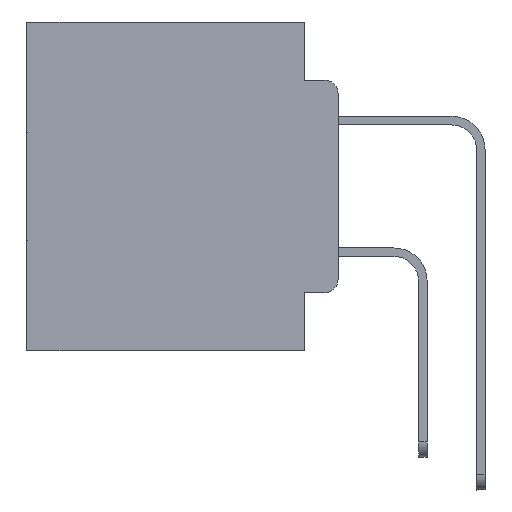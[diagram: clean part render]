
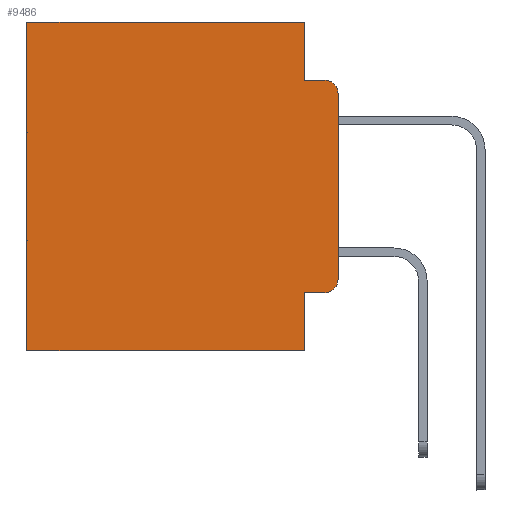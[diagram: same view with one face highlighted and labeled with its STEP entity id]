
A CAD part, left-side view. The second image highlights one B-rep face of the part: STEP entity #9486.
In plain terms, the highlighted planar face has unit normal (-1, 0, 0).
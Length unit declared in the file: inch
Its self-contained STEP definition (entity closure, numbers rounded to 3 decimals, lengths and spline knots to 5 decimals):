
#367 = VERTEX_POINT ( 'NONE', #19383 ) ;
#845 = EDGE_CURVE ( 'NONE', #2925, #9180, #17679, .T. ) ;
#854 = EDGE_CURVE ( 'NONE', #32254, #20370, #29934, .T. ) ;
#862 = LINE ( 'NONE', #9563, #12918 ) ;
#892 = VERTEX_POINT ( 'NONE', #26301 ) ;
#1207 = VECTOR ( 'NONE', #10588, 39.37008 ) ;
#1329 = ORIENTED_EDGE ( 'NONE', *, *, #17962, .F. ) ;
#1883 = DIRECTION ( 'NONE',  ( 0., -1., 0. ) ) ;
#1954 = VECTOR ( 'NONE', #5000, 39.37008 ) ;
#2442 = CARTESIAN_POINT ( 'NONE',  ( 0.298, 0.473, -0.5 ) ) ;
#2782 = DIRECTION ( 'NONE',  ( 0., -1., 0. ) ) ;
#2925 = VERTEX_POINT ( 'NONE', #21016 ) ;
#3417 = LINE ( 'NONE', #28388, #29253 ) ;
#4177 = ORIENTED_EDGE ( 'NONE', *, *, #854, .T. ) ;
#4811 = VERTEX_POINT ( 'NONE', #13942 ) ;
#5000 = DIRECTION ( 'NONE',  ( 0., 0., -1. ) ) ;
#5008 = VECTOR ( 'NONE', #2782, 39.37008 ) ;
#5489 = CARTESIAN_POINT ( 'NONE',  ( 0.298, 0.051, -0.0885 ) ) ;
#6349 = VERTEX_POINT ( 'NONE', #2442 ) ;
#6667 = ORIENTED_EDGE ( 'NONE', *, *, #23556, .F. ) ;
#6783 = VERTEX_POINT ( 'NONE', #32305 ) ;
#6840 = CIRCLE ( 'NONE', #26290, 0.02 ) ;
#7419 = PLANE ( 'NONE',  #22958 ) ;
#7638 = CARTESIAN_POINT ( 'NONE',  ( 0.298, 0.02, -0.1085 ) ) ;
#8050 = CARTESIAN_POINT ( 'NONE',  ( 0.298, 0.473, 0. ) ) ;
#8959 = CIRCLE ( 'NONE', #24914, 0.02 ) ;
#9180 = VERTEX_POINT ( 'NONE', #11302 ) ;
#9474 = VERTEX_POINT ( 'NONE', #12379 ) ;
#9486 = ADVANCED_FACE ( 'NONE', ( #20985 ), #7419, .F. ) ;
#9517 = EDGE_CURVE ( 'NONE', #4811, #9180, #6840, .T. ) ;
#9563 = CARTESIAN_POINT ( 'NONE',  ( 0.298, 0.051, -0.4115 ) ) ;
#10175 = DIRECTION ( 'NONE',  ( 0., 0., -1. ) ) ;
#10588 = DIRECTION ( 'NONE',  ( 0., 0., -1. ) ) ;
#11046 = DIRECTION ( 'NONE',  ( 0., 0., -1. ) ) ;
#11302 = CARTESIAN_POINT ( 'NONE',  ( 0.298, 0.02, -0.0885 ) ) ;
#11827 = ORIENTED_EDGE ( 'NONE', *, *, #845, .F. ) ;
#12379 = CARTESIAN_POINT ( 'NONE',  ( 0.298, 0., -0.3915 ) ) ;
#12559 = ORIENTED_EDGE ( 'NONE', *, *, #31644, .F. ) ;
#12708 = EDGE_CURVE ( 'NONE', #367, #6349, #25029, .T. ) ;
#12726 = DIRECTION ( 'NONE',  ( 0., 0., -1. ) ) ;
#12918 = VECTOR ( 'NONE', #1883, 39.37008 ) ;
#13528 = EDGE_CURVE ( 'NONE', #892, #9474, #8959, .T. ) ;
#13818 = CARTESIAN_POINT ( 'NONE',  ( 0.298, 0., -0.5 ) ) ;
#13942 = CARTESIAN_POINT ( 'NONE',  ( 0.298, 0., -0.1085 ) ) ;
#14646 = DIRECTION ( 'NONE',  ( -1., 0., 0. ) ) ;
#15229 = EDGE_CURVE ( 'NONE', #6783, #892, #862, .T. ) ;
#16896 = VECTOR ( 'NONE', #26852, 39.37008 ) ;
#17547 = DIRECTION ( 'NONE',  ( 0., 0., -1. ) ) ;
#17679 = LINE ( 'NONE', #5489, #5008 ) ;
#17962 = EDGE_CURVE ( 'NONE', #4811, #9474, #28669, .T. ) ;
#18443 = VECTOR ( 'NONE', #31019, 39.37008 ) ;
#19383 = CARTESIAN_POINT ( 'NONE',  ( 0.298, 0.051, -0.5 ) ) ;
#19704 = ORIENTED_EDGE ( 'NONE', *, *, #15229, .T. ) ;
#20111 = CARTESIAN_POINT ( 'NONE',  ( 0.298, 0., 0. ) ) ;
#20180 = VECTOR ( 'NONE', #12726, 39.37008 ) ;
#20370 = VERTEX_POINT ( 'NONE', #27087 ) ;
#20567 = CARTESIAN_POINT ( 'NONE',  ( 0.298, 0.051, 0. ) ) ;
#20780 = ORIENTED_EDGE ( 'NONE', *, *, #26850, .T. ) ;
#20985 = FACE_OUTER_BOUND ( 'NONE', #24886, .T. ) ;
#21016 = CARTESIAN_POINT ( 'NONE',  ( 0.298, 0.051, -0.0885 ) ) ;
#21462 = LINE ( 'NONE', #8050, #1207 ) ;
#21751 = LINE ( 'NONE', #29983, #20180 ) ;
#22958 = AXIS2_PLACEMENT_3D ( 'NONE', #24921, #32162, #17547 ) ;
#23556 = EDGE_CURVE ( 'NONE', #6783, #367, #3417, .T. ) ;
#23867 = ORIENTED_EDGE ( 'NONE', *, *, #9517, .T. ) ;
#24886 = EDGE_LOOP ( 'NONE', ( #1329, #23867, #11827, #12559, #4177, #20780, #29985, #6667, #19704, #27292 ) ) ;
#24914 = AXIS2_PLACEMENT_3D ( 'NONE', #29405, #14646, #31808 ) ;
#24921 = CARTESIAN_POINT ( 'NONE',  ( 0.298, 0., 0. ) ) ;
#25029 = LINE ( 'NONE', #13818, #18443 ) ;
#25151 = DIRECTION ( 'NONE',  ( -1., 0., 0. ) ) ;
#25353 = CARTESIAN_POINT ( 'NONE',  ( 0.298, 0., 0. ) ) ;
#26290 = AXIS2_PLACEMENT_3D ( 'NONE', #7638, #25151, #10175 ) ;
#26301 = CARTESIAN_POINT ( 'NONE',  ( 0.298, 0.02, -0.4115 ) ) ;
#26850 = EDGE_CURVE ( 'NONE', #20370, #6349, #21462, .T. ) ;
#26852 = DIRECTION ( 'NONE',  ( 0., 1., 0. ) ) ;
#27087 = CARTESIAN_POINT ( 'NONE',  ( 0.298, 0.473, 0. ) ) ;
#27292 = ORIENTED_EDGE ( 'NONE', *, *, #13528, .T. ) ;
#28388 = CARTESIAN_POINT ( 'NONE',  ( 0.298, 0.051, 0. ) ) ;
#28669 = LINE ( 'NONE', #20111, #1954 ) ;
#29253 = VECTOR ( 'NONE', #11046, 39.37008 ) ;
#29405 = CARTESIAN_POINT ( 'NONE',  ( 0.298, 0.02, -0.3915 ) ) ;
#29934 = LINE ( 'NONE', #25353, #16896 ) ;
#29983 = CARTESIAN_POINT ( 'NONE',  ( 0.298, 0.051, 0. ) ) ;
#29985 = ORIENTED_EDGE ( 'NONE', *, *, #12708, .F. ) ;
#31019 = DIRECTION ( 'NONE',  ( 0., 1., 0. ) ) ;
#31644 = EDGE_CURVE ( 'NONE', #32254, #2925, #21751, .T. ) ;
#31808 = DIRECTION ( 'NONE',  ( 0., 0., -1. ) ) ;
#32162 = DIRECTION ( 'NONE',  ( 1., 0., 0. ) ) ;
#32254 = VERTEX_POINT ( 'NONE', #20567 ) ;
#32305 = CARTESIAN_POINT ( 'NONE',  ( 0.298, 0.051, -0.4115 ) ) ;
